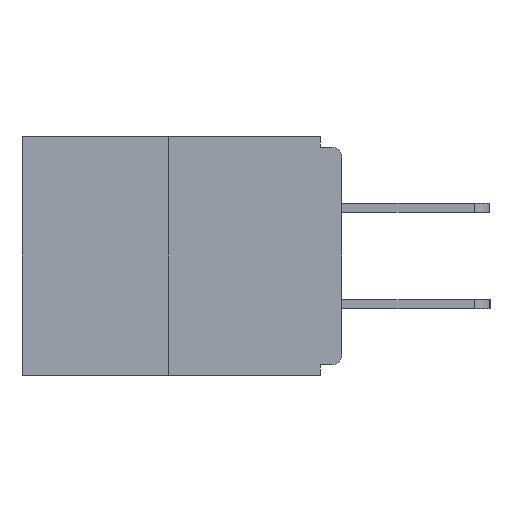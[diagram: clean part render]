
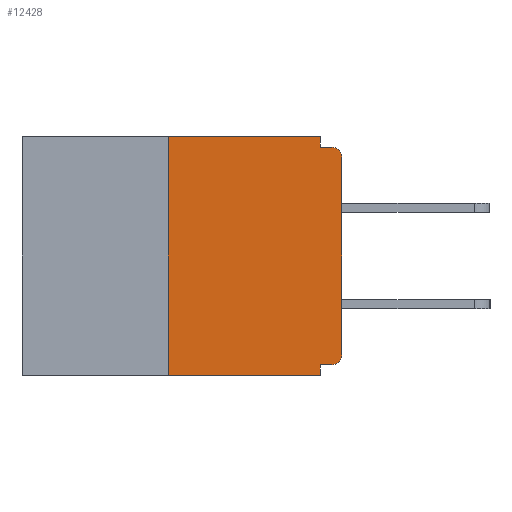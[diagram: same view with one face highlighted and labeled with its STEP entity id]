
A CAD part, left-side view. The second image highlights one B-rep face of the part: STEP entity #12428.
In plain terms, the highlighted planar face has unit normal (-1, 0, 0).
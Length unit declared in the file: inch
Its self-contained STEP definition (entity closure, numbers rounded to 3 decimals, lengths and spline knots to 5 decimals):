
#49 = EDGE_CURVE ( 'NONE', #11979, #227, #1825, .T. ) ;
#227 = VERTEX_POINT ( 'NONE', #10177 ) ;
#461 = LINE ( 'NONE', #12491, #7537 ) ;
#575 = VECTOR ( 'NONE', #8094, 39.37008 ) ;
#585 = DIRECTION ( 'NONE',  ( 0., 0., 1. ) ) ;
#837 = VERTEX_POINT ( 'NONE', #4191 ) ;
#894 = AXIS2_PLACEMENT_3D ( 'NONE', #9892, #1054, #11948 ) ;
#983 = CARTESIAN_POINT ( 'NONE',  ( 0., 0.031, -0.343 ) ) ;
#1021 = ORIENTED_EDGE ( 'NONE', *, *, #11401, .F. ) ;
#1054 = DIRECTION ( 'NONE',  ( -1., 0., 0. ) ) ;
#1193 = DIRECTION ( 'NONE',  ( -1., 0., 0. ) ) ;
#1268 = LINE ( 'NONE', #9997, #12850 ) ;
#1407 = CARTESIAN_POINT ( 'NONE',  ( 0., 0.46, 0. ) ) ;
#1473 = CARTESIAN_POINT ( 'NONE',  ( 0., 0., -0.313 ) ) ;
#1500 = DIRECTION ( 'NONE',  ( 1., 0., 0. ) ) ;
#1778 = VERTEX_POINT ( 'NONE', #2474 ) ;
#1825 = LINE ( 'NONE', #9161, #8294 ) ;
#1833 = ORIENTED_EDGE ( 'NONE', *, *, #11512, .F. ) ;
#1974 = LINE ( 'NONE', #983, #10157 ) ;
#2104 = ORIENTED_EDGE ( 'NONE', *, *, #2676, .F. ) ;
#2464 = CARTESIAN_POINT ( 'NONE',  ( 0., 0., -0.328 ) ) ;
#2474 = CARTESIAN_POINT ( 'NONE',  ( 0., 0.031, -0.015 ) ) ;
#2481 = CARTESIAN_POINT ( 'NONE',  ( 0., 0., -0.03 ) ) ;
#2676 = EDGE_CURVE ( 'NONE', #1778, #2884, #8761, .T. ) ;
#2884 = VERTEX_POINT ( 'NONE', #8707 ) ;
#3039 = ORIENTED_EDGE ( 'NONE', *, *, #8982, .T. ) ;
#3263 = VECTOR ( 'NONE', #13389, 39.37008 ) ;
#3350 = EDGE_LOOP ( 'NONE', ( #10053, #12602, #3039, #12836, #1021, #12348, #11132, #10046, #2104, #1833 ) ) ;
#3460 = AXIS2_PLACEMENT_3D ( 'NONE', #7686, #1193, #8804 ) ;
#3472 = PLANE ( 'NONE',  #12727 ) ;
#3638 = CARTESIAN_POINT ( 'NONE',  ( 0., 0.031, 0. ) ) ;
#3774 = LINE ( 'NONE', #11848, #5283 ) ;
#4191 = CARTESIAN_POINT ( 'NONE',  ( 0., 0.015, -0.328 ) ) ;
#4905 = FACE_OUTER_BOUND ( 'NONE', #3350, .T. ) ;
#4972 = DIRECTION ( 'NONE',  ( 0., 0., -1. ) ) ;
#5283 = VECTOR ( 'NONE', #12927, 39.37008 ) ;
#5341 = EDGE_CURVE ( 'NONE', #7711, #6112, #1974, .T. ) ;
#5872 = DIRECTION ( 'NONE',  ( 0., -1., 0. ) ) ;
#6035 = CARTESIAN_POINT ( 'NONE',  ( 0., 0., -0.015 ) ) ;
#6112 = VERTEX_POINT ( 'NONE', #13053 ) ;
#6246 = EDGE_CURVE ( 'NONE', #6599, #8413, #461, .T. ) ;
#6511 = VERTEX_POINT ( 'NONE', #3638 ) ;
#6599 = VERTEX_POINT ( 'NONE', #1473 ) ;
#7005 = LINE ( 'NONE', #2464, #3263 ) ;
#7537 = VECTOR ( 'NONE', #585, 39.37008 ) ;
#7686 = CARTESIAN_POINT ( 'NONE',  ( 0., 0.015, -0.313 ) ) ;
#7711 = VERTEX_POINT ( 'NONE', #9391 ) ;
#8061 = VECTOR ( 'NONE', #10245, 39.37008 ) ;
#8094 = DIRECTION ( 'NONE',  ( 0., -1., 0. ) ) ;
#8174 = LINE ( 'NONE', #9071, #575 ) ;
#8294 = VECTOR ( 'NONE', #10401, 39.37008 ) ;
#8413 = VERTEX_POINT ( 'NONE', #2481 ) ;
#8626 = CARTESIAN_POINT ( 'NONE',  ( 0., 0.25, -0.343 ) ) ;
#8707 = CARTESIAN_POINT ( 'NONE',  ( 0., 0.015, -0.015 ) ) ;
#8761 = LINE ( 'NONE', #6035, #8061 ) ;
#8762 = CIRCLE ( 'NONE', #3460, 0.015 ) ;
#8804 = DIRECTION ( 'NONE',  ( 0., 0., -1. ) ) ;
#8982 = EDGE_CURVE ( 'NONE', #11979, #6112, #8174, .T. ) ;
#9071 = CARTESIAN_POINT ( 'NONE',  ( 0., 0.46, -0.343 ) ) ;
#9161 = CARTESIAN_POINT ( 'NONE',  ( 0., 0.25, 0. ) ) ;
#9391 = CARTESIAN_POINT ( 'NONE',  ( 0., 0.031, -0.328 ) ) ;
#9534 = EDGE_CURVE ( 'NONE', #837, #6599, #8762, .T. ) ;
#9892 = CARTESIAN_POINT ( 'NONE',  ( 0., 0.015, -0.03 ) ) ;
#9997 = CARTESIAN_POINT ( 'NONE',  ( 0., 0.46, 0. ) ) ;
#10046 = ORIENTED_EDGE ( 'NONE', *, *, #13119, .T. ) ;
#10053 = ORIENTED_EDGE ( 'NONE', *, *, #10288, .F. ) ;
#10157 = VECTOR ( 'NONE', #11915, 39.37008 ) ;
#10177 = CARTESIAN_POINT ( 'NONE',  ( 0., 0.25, 0. ) ) ;
#10245 = DIRECTION ( 'NONE',  ( 0., -1., 0. ) ) ;
#10288 = EDGE_CURVE ( 'NONE', #227, #6511, #1268, .T. ) ;
#10401 = DIRECTION ( 'NONE',  ( 0., 0., 1. ) ) ;
#11132 = ORIENTED_EDGE ( 'NONE', *, *, #6246, .T. ) ;
#11401 = EDGE_CURVE ( 'NONE', #837, #7711, #7005, .T. ) ;
#11512 = EDGE_CURVE ( 'NONE', #6511, #1778, #3774, .T. ) ;
#11848 = CARTESIAN_POINT ( 'NONE',  ( 0., 0.031, 0. ) ) ;
#11915 = DIRECTION ( 'NONE',  ( 0., 0., -1. ) ) ;
#11948 = DIRECTION ( 'NONE',  ( 0., 0., -1. ) ) ;
#11979 = VERTEX_POINT ( 'NONE', #8626 ) ;
#12348 = ORIENTED_EDGE ( 'NONE', *, *, #9534, .T. ) ;
#12428 = ADVANCED_FACE ( 'NONE', ( #4905 ), #3472, .F. ) ;
#12491 = CARTESIAN_POINT ( 'NONE',  ( 0., 0., 0. ) ) ;
#12602 = ORIENTED_EDGE ( 'NONE', *, *, #49, .F. ) ;
#12727 = AXIS2_PLACEMENT_3D ( 'NONE', #1407, #1500, #4972 ) ;
#12836 = ORIENTED_EDGE ( 'NONE', *, *, #5341, .F. ) ;
#12850 = VECTOR ( 'NONE', #5872, 39.37008 ) ;
#12927 = DIRECTION ( 'NONE',  ( 0., 0., -1. ) ) ;
#13053 = CARTESIAN_POINT ( 'NONE',  ( 0., 0.031, -0.343 ) ) ;
#13119 = EDGE_CURVE ( 'NONE', #8413, #2884, #13985, .T. ) ;
#13389 = DIRECTION ( 'NONE',  ( 0., 1., 0. ) ) ;
#13985 = CIRCLE ( 'NONE', #894, 0.015 ) ;
